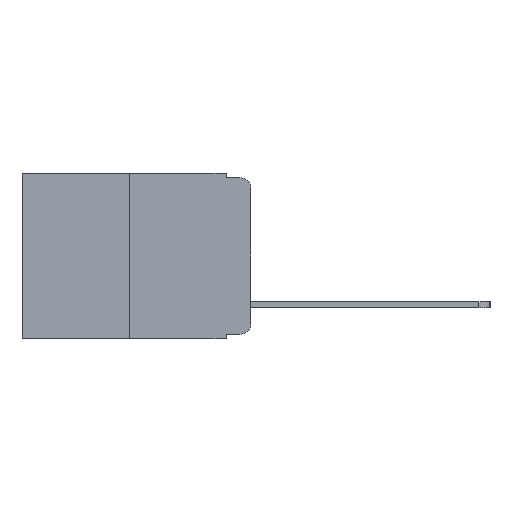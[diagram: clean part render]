
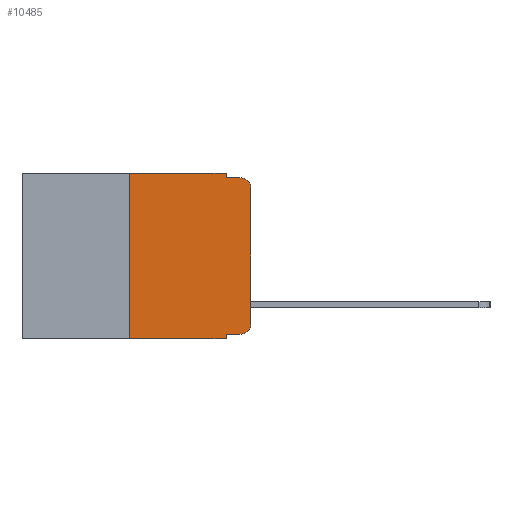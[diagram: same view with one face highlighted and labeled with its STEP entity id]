
A CAD part, left-side view. The second image highlights one B-rep face of the part: STEP entity #10485.
In plain terms, the highlighted planar face has unit normal (-1, 0, 0).
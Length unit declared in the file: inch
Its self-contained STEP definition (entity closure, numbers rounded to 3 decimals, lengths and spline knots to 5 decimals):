
#25 = CIRCLE ( 'NONE', #9642, 0.02 ) ;
#505 = DIRECTION ( 'NONE',  ( 0., 0., -1. ) ) ;
#870 = VERTEX_POINT ( 'NONE', #4665 ) ;
#1188 = VERTEX_POINT ( 'NONE', #5345 ) ;
#1274 = DIRECTION ( 'NONE',  ( 1., 0., 0. ) ) ;
#1369 = EDGE_CURVE ( 'NONE', #6446, #10340, #10598, .T. ) ;
#1554 = EDGE_CURVE ( 'NONE', #6446, #11331, #6267, .T. ) ;
#1556 = EDGE_CURVE ( 'NONE', #11331, #5009, #25, .T. ) ;
#1677 = DIRECTION ( 'NONE',  ( 0., -1., 0. ) ) ;
#1728 = CARTESIAN_POINT ( 'NONE',  ( 0., 0.473, 0. ) ) ;
#1844 = VECTOR ( 'NONE', #9738, 39.37008 ) ;
#1911 = VERTEX_POINT ( 'NONE', #2530 ) ;
#1926 = AXIS2_PLACEMENT_3D ( 'NONE', #2467, #1274, #8740 ) ;
#2106 = EDGE_CURVE ( 'NONE', #870, #10340, #11733, .T. ) ;
#2273 = EDGE_CURVE ( 'NONE', #5009, #10621, #2579, .T. ) ;
#2290 = EDGE_CURVE ( 'NONE', #10621, #5511, #5193, .T. ) ;
#2295 = EDGE_CURVE ( 'NONE', #1911, #5511, #4857, .T. ) ;
#2313 = EDGE_CURVE ( 'NONE', #870, #7957, #12018, .T. ) ;
#2338 = EDGE_CURVE ( 'NONE', #1188, #1911, #11480, .T. ) ;
#2467 = CARTESIAN_POINT ( 'NONE',  ( 0., 0.473, 0. ) ) ;
#2530 = CARTESIAN_POINT ( 'NONE',  ( 0., 0.051, -0.01 ) ) ;
#2579 = LINE ( 'NONE', #9132, #7938 ) ;
#2683 = DIRECTION ( 'NONE',  ( 0., 0., -1. ) ) ;
#2977 = EDGE_CURVE ( 'NONE', #7957, #1188, #10785, .T. ) ;
#3056 = DIRECTION ( 'NONE',  ( 0., 0., 1. ) ) ;
#4665 = CARTESIAN_POINT ( 'NONE',  ( 0., 0.25, -0.343 ) ) ;
#4857 = LINE ( 'NONE', #11475, #1844 ) ;
#5009 = VERTEX_POINT ( 'NONE', #9000 ) ;
#5122 = AXIS2_PLACEMENT_3D ( 'NONE', #5690, #5649, #505 ) ;
#5175 = CARTESIAN_POINT ( 'NONE',  ( 0., 0.25, 0. ) ) ;
#5193 = CIRCLE ( 'NONE', #5122, 0.02 ) ;
#5345 = CARTESIAN_POINT ( 'NONE',  ( 0., 0.051, 0. ) ) ;
#5494 = EDGE_LOOP ( 'NONE', ( #9878, #12850, #11535, #8998, #8004, #7916, #7497, #6760, #6644, #6351 ) ) ;
#5511 = VERTEX_POINT ( 'NONE', #8177 ) ;
#5649 = DIRECTION ( 'NONE',  ( -1., 0., 0. ) ) ;
#5690 = CARTESIAN_POINT ( 'NONE',  ( 0., 0.02, -0.03 ) ) ;
#6201 = VECTOR ( 'NONE', #1677, 39.37008 ) ;
#6267 = LINE ( 'NONE', #12758, #10837 ) ;
#6351 = ORIENTED_EDGE ( 'NONE', *, *, #1556, .T. ) ;
#6446 = VERTEX_POINT ( 'NONE', #6761 ) ;
#6644 = ORIENTED_EDGE ( 'NONE', *, *, #1554, .T. ) ;
#6760 = ORIENTED_EDGE ( 'NONE', *, *, #1369, .F. ) ;
#6761 = CARTESIAN_POINT ( 'NONE',  ( 0., 0.051, -0.333 ) ) ;
#6840 = DIRECTION ( 'NONE',  ( 0., -1., 0. ) ) ;
#7355 = VECTOR ( 'NONE', #3056, 39.37008 ) ;
#7364 = CARTESIAN_POINT ( 'NONE',  ( 0., 0.25, 0. ) ) ;
#7370 = VECTOR ( 'NONE', #7734, 39.37008 ) ;
#7449 = DIRECTION ( 'NONE',  ( 0., 0., 1. ) ) ;
#7497 = ORIENTED_EDGE ( 'NONE', *, *, #2106, .T. ) ;
#7700 = VECTOR ( 'NONE', #8222, 39.37008 ) ;
#7734 = DIRECTION ( 'NONE',  ( 0., -1., 0. ) ) ;
#7916 = ORIENTED_EDGE ( 'NONE', *, *, #2313, .F. ) ;
#7938 = VECTOR ( 'NONE', #7449, 39.37008 ) ;
#7957 = VERTEX_POINT ( 'NONE', #5175 ) ;
#8004 = ORIENTED_EDGE ( 'NONE', *, *, #2977, .F. ) ;
#8177 = CARTESIAN_POINT ( 'NONE',  ( 0., 0.02, -0.01 ) ) ;
#8222 = DIRECTION ( 'NONE',  ( 0., 0., -1. ) ) ;
#8399 = CARTESIAN_POINT ( 'NONE',  ( 0., 0.051, 0. ) ) ;
#8740 = DIRECTION ( 'NONE',  ( 0., 0., -1. ) ) ;
#8998 = ORIENTED_EDGE ( 'NONE', *, *, #2338, .F. ) ;
#9000 = CARTESIAN_POINT ( 'NONE',  ( 0., 0., -0.313 ) ) ;
#9132 = CARTESIAN_POINT ( 'NONE',  ( 0., 0., 0. ) ) ;
#9183 = VECTOR ( 'NONE', #2683, 39.37008 ) ;
#9642 = AXIS2_PLACEMENT_3D ( 'NONE', #12347, #12319, #12233 ) ;
#9738 = DIRECTION ( 'NONE',  ( 0., -1., 0. ) ) ;
#9878 = ORIENTED_EDGE ( 'NONE', *, *, #2273, .T. ) ;
#10340 = VERTEX_POINT ( 'NONE', #10611 ) ;
#10403 = FACE_OUTER_BOUND ( 'NONE', #5494, .T. ) ;
#10485 = ADVANCED_FACE ( 'NONE', ( #10403 ), #11293, .F. ) ;
#10598 = LINE ( 'NONE', #11158, #7700 ) ;
#10611 = CARTESIAN_POINT ( 'NONE',  ( 0., 0.051, -0.343 ) ) ;
#10621 = VERTEX_POINT ( 'NONE', #11645 ) ;
#10785 = LINE ( 'NONE', #1728, #6201 ) ;
#10837 = VECTOR ( 'NONE', #6840, 39.37008 ) ;
#11158 = CARTESIAN_POINT ( 'NONE',  ( 0., 0.051, 0. ) ) ;
#11293 = PLANE ( 'NONE',  #1926 ) ;
#11331 = VERTEX_POINT ( 'NONE', #11462 ) ;
#11462 = CARTESIAN_POINT ( 'NONE',  ( 0., 0.02, -0.333 ) ) ;
#11475 = CARTESIAN_POINT ( 'NONE',  ( 0., 0.051, -0.01 ) ) ;
#11480 = LINE ( 'NONE', #8399, #9183 ) ;
#11535 = ORIENTED_EDGE ( 'NONE', *, *, #2295, .F. ) ;
#11645 = CARTESIAN_POINT ( 'NONE',  ( 0., 0., -0.03 ) ) ;
#11733 = LINE ( 'NONE', #12333, #7370 ) ;
#12018 = LINE ( 'NONE', #7364, #7355 ) ;
#12233 = DIRECTION ( 'NONE',  ( 0., 0., -1. ) ) ;
#12319 = DIRECTION ( 'NONE',  ( -1., 0., 0. ) ) ;
#12333 = CARTESIAN_POINT ( 'NONE',  ( 0., 0.473, -0.343 ) ) ;
#12347 = CARTESIAN_POINT ( 'NONE',  ( 0., 0.02, -0.313 ) ) ;
#12758 = CARTESIAN_POINT ( 'NONE',  ( 0., 0.051, -0.333 ) ) ;
#12850 = ORIENTED_EDGE ( 'NONE', *, *, #2290, .T. ) ;
